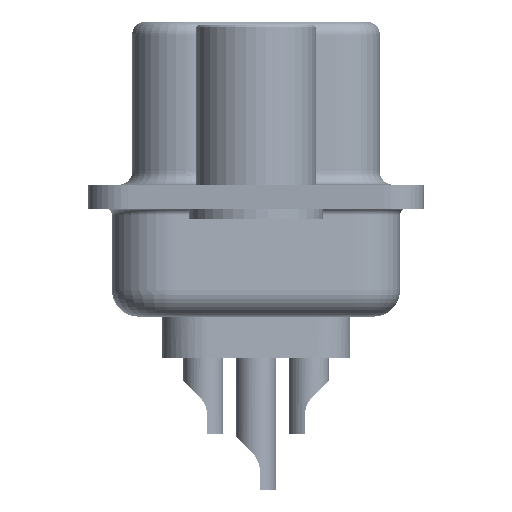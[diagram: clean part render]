
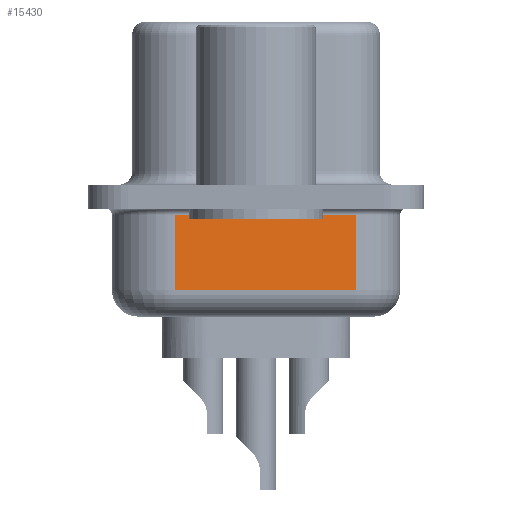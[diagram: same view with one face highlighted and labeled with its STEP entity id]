
A CAD part, left-side view. The second image highlights one B-rep face of the part: STEP entity #15430.
In plain terms, the highlighted planar face has unit normal (-0.985, -0.174, 0).
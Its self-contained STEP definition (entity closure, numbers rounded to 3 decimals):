
#114 = ORIENTED_EDGE ( 'NONE', *, *, #2318, .T. ) ;
#1017 = LINE ( 'NONE', #23428, #8548 ) ;
#2153 = LINE ( 'NONE', #13351, #4038 ) ;
#2318 = EDGE_CURVE ( 'NONE', #33404, #10308, #1017, .T. ) ;
#2374 = CARTESIAN_POINT ( 'NONE',  ( 3.13, 3.053, -3.5 ) ) ;
#4038 = VECTOR ( 'NONE', #35241, 1000. ) ;
#4117 = VECTOR ( 'NONE', #19490, 1000. ) ;
#4808 = CARTESIAN_POINT ( 'NONE',  ( 3.13, 3.053, -4.5 ) ) ;
#5148 = EDGE_CURVE ( 'NONE', #13551, #10307, #2153, .T. ) ;
#6779 = CARTESIAN_POINT ( 'NONE',  ( 3.13, 3.053, -3.5 ) ) ;
#6833 = ORIENTED_EDGE ( 'NONE', *, *, #6871, .T. ) ;
#6871 = EDGE_CURVE ( 'NONE', #13551, #33404, #12262, .T. ) ;
#7523 = EDGE_CURVE ( 'NONE', #10308, #10307, #25020, .T. ) ;
#8305 = CARTESIAN_POINT ( 'NONE',  ( 3.13, 3.053, -0.7 ) ) ;
#8548 = VECTOR ( 'NONE', #15315, 1000. ) ;
#10151 = AXIS2_PLACEMENT_3D ( 'NONE', #4808, #21165, #26323 ) ;
#10307 = VERTEX_POINT ( 'NONE', #35376 ) ;
#10308 = VERTEX_POINT ( 'NONE', #27490 ) ;
#12262 = LINE ( 'NONE', #6779, #18692 ) ;
#13351 = CARTESIAN_POINT ( 'NONE',  ( 3.13, 3.053, -4.5 ) ) ;
#13551 = VERTEX_POINT ( 'NONE', #2374 ) ;
#15315 = DIRECTION ( 'NONE',  ( 0., 0., 1. ) ) ;
#15430 = ADVANCED_FACE ( 'NONE', ( #23920 ), #15813, .F. ) ;
#15813 = PLANE ( 'NONE',  #10151 ) ;
#18692 = VECTOR ( 'NONE', #23844, 1000. ) ;
#19490 = DIRECTION ( 'NONE',  ( -0.174, 0.985, 0. ) ) ;
#20395 = ORIENTED_EDGE ( 'NONE', *, *, #7523, .T. ) ;
#21165 = DIRECTION ( 'NONE',  ( 0.985, 0.174, 0. ) ) ;
#22757 = ORIENTED_EDGE ( 'NONE', *, *, #5148, .F. ) ;
#23428 = CARTESIAN_POINT ( 'NONE',  ( 4.329, -3.747, -4.5 ) ) ;
#23844 = DIRECTION ( 'NONE',  ( 0.174, -0.985, 0. ) ) ;
#23920 = FACE_OUTER_BOUND ( 'NONE', #28750, .T. ) ;
#25020 = LINE ( 'NONE', #8305, #4117 ) ;
#26323 = DIRECTION ( 'NONE',  ( -0.174, 0.985, 0. ) ) ;
#27490 = CARTESIAN_POINT ( 'NONE',  ( 4.329, -3.747, -0.7 ) ) ;
#28750 = EDGE_LOOP ( 'NONE', ( #22757, #6833, #114, #20395 ) ) ;
#31685 = CARTESIAN_POINT ( 'NONE',  ( 4.329, -3.747, -3.5 ) ) ;
#33404 = VERTEX_POINT ( 'NONE', #31685 ) ;
#35241 = DIRECTION ( 'NONE',  ( 0., 0., 1. ) ) ;
#35376 = CARTESIAN_POINT ( 'NONE',  ( 3.13, 3.053, -0.7 ) ) ;
